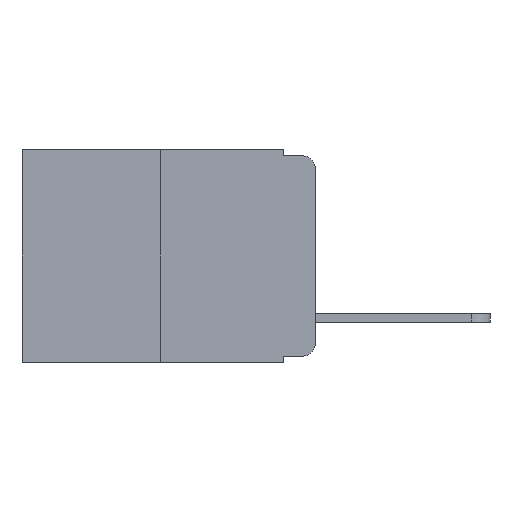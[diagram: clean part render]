
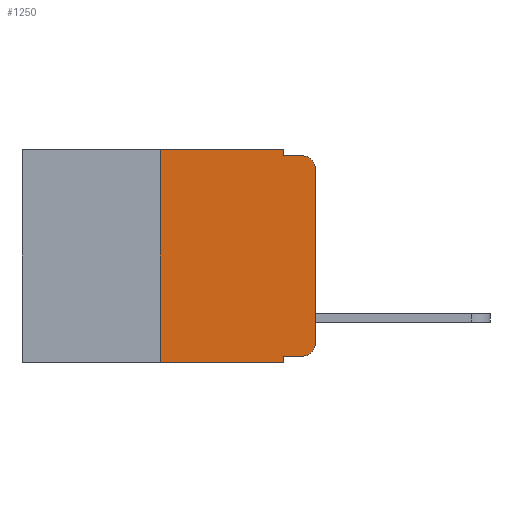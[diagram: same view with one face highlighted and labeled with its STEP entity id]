
A CAD part, left-side view. The second image highlights one B-rep face of the part: STEP entity #1250.
In plain terms, the highlighted planar face has unit normal (-1, 0, 0).
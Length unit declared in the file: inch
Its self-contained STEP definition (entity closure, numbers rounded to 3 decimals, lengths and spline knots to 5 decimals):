
#45 = PLANE ( 'NONE',  #5185 ) ;
#343 = FACE_OUTER_BOUND ( 'NONE', #3693, .T. ) ;
#597 = CARTESIAN_POINT ( 'NONE',  ( 0., 0., -0.03 ) ) ;
#618 = CARTESIAN_POINT ( 'NONE',  ( 0., 0.02, -0.333 ) ) ;
#666 = VERTEX_POINT ( 'NONE', #3274 ) ;
#743 = EDGE_CURVE ( 'NONE', #2015, #9847, #6347, .T. ) ;
#1088 = VERTEX_POINT ( 'NONE', #10145 ) ;
#1196 = LINE ( 'NONE', #6308, #5250 ) ;
#1250 = ADVANCED_FACE ( 'NONE', ( #343 ), #45, .F. ) ;
#1281 = LINE ( 'NONE', #2403, #1559 ) ;
#1540 = CARTESIAN_POINT ( 'NONE',  ( 0., 0.25, 0. ) ) ;
#1559 = VECTOR ( 'NONE', #2424, 39.37008 ) ;
#2015 = VERTEX_POINT ( 'NONE', #7700 ) ;
#2022 = VERTEX_POINT ( 'NONE', #5577 ) ;
#2266 = DIRECTION ( 'NONE',  ( 0., -1., 0. ) ) ;
#2403 = CARTESIAN_POINT ( 'NONE',  ( 0., 0.473, -0.343 ) ) ;
#2424 = DIRECTION ( 'NONE',  ( 0., -1., 0. ) ) ;
#2686 = LINE ( 'NONE', #6777, #8491 ) ;
#3164 = LINE ( 'NONE', #8585, #8916 ) ;
#3274 = CARTESIAN_POINT ( 'NONE',  ( 0., 0.051, -0.343 ) ) ;
#3680 = CARTESIAN_POINT ( 'NONE',  ( 0., 0.25, -0.343 ) ) ;
#3693 = EDGE_LOOP ( 'NONE', ( #7940, #7948, #8459, #8646, #8873, #8979, #9104, #9210, #9548, #9657 ) ) ;
#3741 = EDGE_CURVE ( 'NONE', #6844, #2022, #4506, .T. ) ;
#3798 = DIRECTION ( 'NONE',  ( 0., -1., 0. ) ) ;
#3880 = VECTOR ( 'NONE', #8121, 39.37008 ) ;
#4214 = CIRCLE ( 'NONE', #9259, 0.02 ) ;
#4506 = CIRCLE ( 'NONE', #5335, 0.02 ) ;
#4551 = EDGE_CURVE ( 'NONE', #4849, #2015, #6031, .T. ) ;
#4644 = VERTEX_POINT ( 'NONE', #3680 ) ;
#4849 = VERTEX_POINT ( 'NONE', #1540 ) ;
#4949 = VERTEX_POINT ( 'NONE', #597 ) ;
#5185 = AXIS2_PLACEMENT_3D ( 'NONE', #10014, #7803, #7788 ) ;
#5250 = VECTOR ( 'NONE', #8486, 39.37008 ) ;
#5335 = AXIS2_PLACEMENT_3D ( 'NONE', #9717, #10109, #10105 ) ;
#5576 = EDGE_CURVE ( 'NONE', #1088, #666, #1196, .T. ) ;
#5577 = CARTESIAN_POINT ( 'NONE',  ( 0., 0., -0.313 ) ) ;
#5665 = CARTESIAN_POINT ( 'NONE',  ( 0., 0.051, -0.01 ) ) ;
#5682 = EDGE_CURVE ( 'NONE', #4949, #8030, #4214, .T. ) ;
#5900 = DIRECTION ( 'NONE',  ( 0., 0., -1. ) ) ;
#6031 = LINE ( 'NONE', #9688, #3880 ) ;
#6271 = DIRECTION ( 'NONE',  ( 0., 0., 1. ) ) ;
#6285 = CARTESIAN_POINT ( 'NONE',  ( 0., 0., 0. ) ) ;
#6308 = CARTESIAN_POINT ( 'NONE',  ( 0., 0.051, 0. ) ) ;
#6347 = LINE ( 'NONE', #6938, #8009 ) ;
#6432 = DIRECTION ( 'NONE',  ( 0., 0., 1. ) ) ;
#6629 = VECTOR ( 'NONE', #6271, 39.37008 ) ;
#6646 = CARTESIAN_POINT ( 'NONE',  ( 0., 0.02, -0.01 ) ) ;
#6777 = CARTESIAN_POINT ( 'NONE',  ( 0., 0.051, -0.01 ) ) ;
#6844 = VERTEX_POINT ( 'NONE', #618 ) ;
#6938 = CARTESIAN_POINT ( 'NONE',  ( 0., 0.051, 0. ) ) ;
#7315 = VECTOR ( 'NONE', #6432, 39.37008 ) ;
#7323 = EDGE_CURVE ( 'NONE', #4644, #666, #1281, .T. ) ;
#7532 = LINE ( 'NONE', #9481, #7315 ) ;
#7700 = CARTESIAN_POINT ( 'NONE',  ( 0., 0.051, 0. ) ) ;
#7788 = DIRECTION ( 'NONE',  ( 0., 0., -1. ) ) ;
#7803 = DIRECTION ( 'NONE',  ( 1., 0., 0. ) ) ;
#7844 = DIRECTION ( 'NONE',  ( -1., 0., 0. ) ) ;
#7869 = CARTESIAN_POINT ( 'NONE',  ( 0., 0.02, -0.03 ) ) ;
#7909 = DIRECTION ( 'NONE',  ( 0., 0., -1. ) ) ;
#7940 = ORIENTED_EDGE ( 'NONE', *, *, #8994, .T. ) ;
#7948 = ORIENTED_EDGE ( 'NONE', *, *, #5682, .T. ) ;
#8009 = VECTOR ( 'NONE', #5900, 39.37008 ) ;
#8030 = VERTEX_POINT ( 'NONE', #6646 ) ;
#8121 = DIRECTION ( 'NONE',  ( 0., -1., 0. ) ) ;
#8458 = EDGE_CURVE ( 'NONE', #1088, #6844, #3164, .T. ) ;
#8459 = ORIENTED_EDGE ( 'NONE', *, *, #8514, .F. ) ;
#8484 = LINE ( 'NONE', #6285, #6629 ) ;
#8486 = DIRECTION ( 'NONE',  ( 0., 0., -1. ) ) ;
#8491 = VECTOR ( 'NONE', #2266, 39.37008 ) ;
#8514 = EDGE_CURVE ( 'NONE', #9847, #8030, #2686, .T. ) ;
#8585 = CARTESIAN_POINT ( 'NONE',  ( 0., 0.051, -0.333 ) ) ;
#8646 = ORIENTED_EDGE ( 'NONE', *, *, #743, .F. ) ;
#8873 = ORIENTED_EDGE ( 'NONE', *, *, #4551, .F. ) ;
#8910 = EDGE_CURVE ( 'NONE', #4644, #4849, #7532, .T. ) ;
#8916 = VECTOR ( 'NONE', #3798, 39.37008 ) ;
#8979 = ORIENTED_EDGE ( 'NONE', *, *, #8910, .F. ) ;
#8994 = EDGE_CURVE ( 'NONE', #2022, #4949, #8484, .T. ) ;
#9104 = ORIENTED_EDGE ( 'NONE', *, *, #7323, .T. ) ;
#9210 = ORIENTED_EDGE ( 'NONE', *, *, #5576, .F. ) ;
#9259 = AXIS2_PLACEMENT_3D ( 'NONE', #7869, #7844, #7909 ) ;
#9481 = CARTESIAN_POINT ( 'NONE',  ( 0., 0.25, 0. ) ) ;
#9548 = ORIENTED_EDGE ( 'NONE', *, *, #8458, .T. ) ;
#9657 = ORIENTED_EDGE ( 'NONE', *, *, #3741, .T. ) ;
#9688 = CARTESIAN_POINT ( 'NONE',  ( 0., 0.473, 0. ) ) ;
#9717 = CARTESIAN_POINT ( 'NONE',  ( 0., 0.02, -0.313 ) ) ;
#9847 = VERTEX_POINT ( 'NONE', #5665 ) ;
#10014 = CARTESIAN_POINT ( 'NONE',  ( 0., 0.473, 0. ) ) ;
#10105 = DIRECTION ( 'NONE',  ( 0., 0., -1. ) ) ;
#10109 = DIRECTION ( 'NONE',  ( -1., 0., 0. ) ) ;
#10145 = CARTESIAN_POINT ( 'NONE',  ( 0., 0.051, -0.333 ) ) ;
